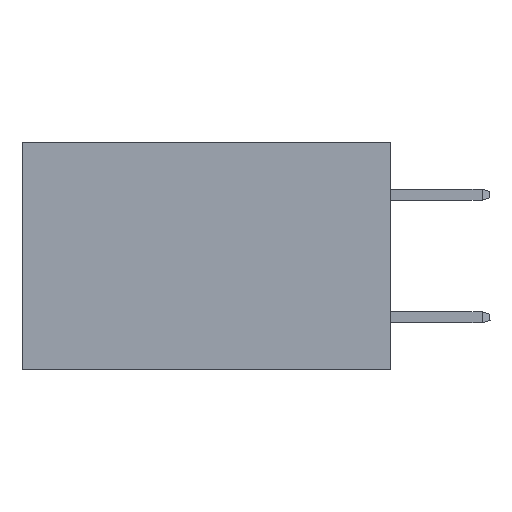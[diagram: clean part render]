
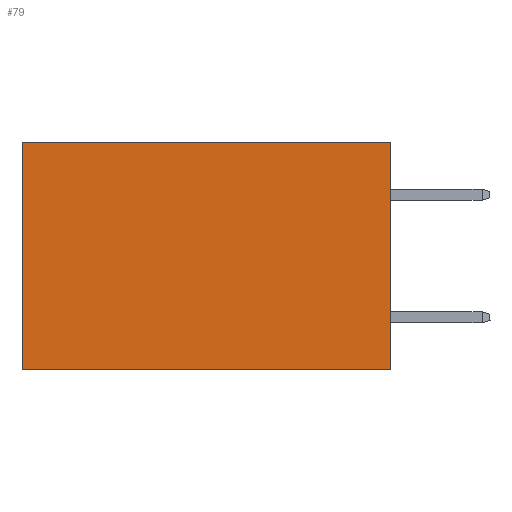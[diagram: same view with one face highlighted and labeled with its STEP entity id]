
A CAD part, left-side view. The second image highlights one B-rep face of the part: STEP entity #79.
In plain terms, the highlighted planar face has unit normal (-1, 0, 0).
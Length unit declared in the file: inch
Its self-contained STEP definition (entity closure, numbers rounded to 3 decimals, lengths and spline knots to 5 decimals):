
#79 = ADVANCED_FACE ( 'NONE', ( #3573 ), #24152, .F. ) ;
#646 = VECTOR ( 'NONE', #1018, 39.37008 ) ;
#721 = CARTESIAN_POINT ( 'NONE',  ( 0.2875, 0.6, 0. ) ) ;
#1018 = DIRECTION ( 'NONE',  ( 0., 1., 0. ) ) ;
#1247 = DIRECTION ( 'NONE',  ( 0., 0., -1. ) ) ;
#3111 = EDGE_LOOP ( 'NONE', ( #23903, #8693, #8407, #7342 ) ) ;
#3573 = FACE_OUTER_BOUND ( 'NONE', #3111, .T. ) ;
#4703 = EDGE_CURVE ( 'NONE', #11004, #15604, #19072, .T. ) ;
#5088 = CARTESIAN_POINT ( 'NONE',  ( 0.2875, 0., -0.37 ) ) ;
#6717 = CARTESIAN_POINT ( 'NONE',  ( 0.2875, 0.6, 0. ) ) ;
#7201 = VECTOR ( 'NONE', #24532, 39.37008 ) ;
#7275 = CARTESIAN_POINT ( 'NONE',  ( 0.2875, 0., -0.37 ) ) ;
#7342 = ORIENTED_EDGE ( 'NONE', *, *, #12550, .T. ) ;
#7737 = DIRECTION ( 'NONE',  ( 0., 0., -1. ) ) ;
#8407 = ORIENTED_EDGE ( 'NONE', *, *, #9583, .F. ) ;
#8543 = LINE ( 'NONE', #721, #7201 ) ;
#8693 = ORIENTED_EDGE ( 'NONE', *, *, #4703, .F. ) ;
#9583 = EDGE_CURVE ( 'NONE', #24539, #11004, #18005, .T. ) ;
#11004 = VERTEX_POINT ( 'NONE', #7275 ) ;
#11400 = CARTESIAN_POINT ( 'NONE',  ( 0.2875, 0., 0. ) ) ;
#12550 = EDGE_CURVE ( 'NONE', #24539, #19899, #23544, .T. ) ;
#12621 = CARTESIAN_POINT ( 'NONE',  ( 0.2875, 0.6, -0.37 ) ) ;
#13939 = DIRECTION ( 'NONE',  ( 1., 0., 0. ) ) ;
#15361 = VECTOR ( 'NONE', #1247, 39.37008 ) ;
#15604 = VERTEX_POINT ( 'NONE', #12621 ) ;
#15750 = DIRECTION ( 'NONE',  ( 0., 1., 0. ) ) ;
#15806 = EDGE_CURVE ( 'NONE', #19899, #15604, #8543, .T. ) ;
#17696 = CARTESIAN_POINT ( 'NONE',  ( 0.2875, 0., 0. ) ) ;
#18005 = LINE ( 'NONE', #11400, #15361 ) ;
#19072 = LINE ( 'NONE', #5088, #646 ) ;
#19899 = VERTEX_POINT ( 'NONE', #6717 ) ;
#22261 = CARTESIAN_POINT ( 'NONE',  ( 0.2875, 0., 0. ) ) ;
#23544 = LINE ( 'NONE', #17696, #24894 ) ;
#23903 = ORIENTED_EDGE ( 'NONE', *, *, #15806, .T. ) ;
#24152 = PLANE ( 'NONE',  #25114 ) ;
#24532 = DIRECTION ( 'NONE',  ( 0., 0., -1. ) ) ;
#24539 = VERTEX_POINT ( 'NONE', #25920 ) ;
#24894 = VECTOR ( 'NONE', #15750, 39.37008 ) ;
#25114 = AXIS2_PLACEMENT_3D ( 'NONE', #22261, #13939, #7737 ) ;
#25920 = CARTESIAN_POINT ( 'NONE',  ( 0.2875, 0., 0. ) ) ;
